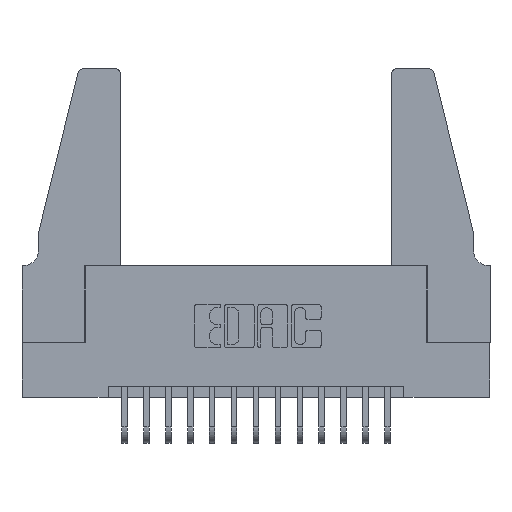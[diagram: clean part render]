
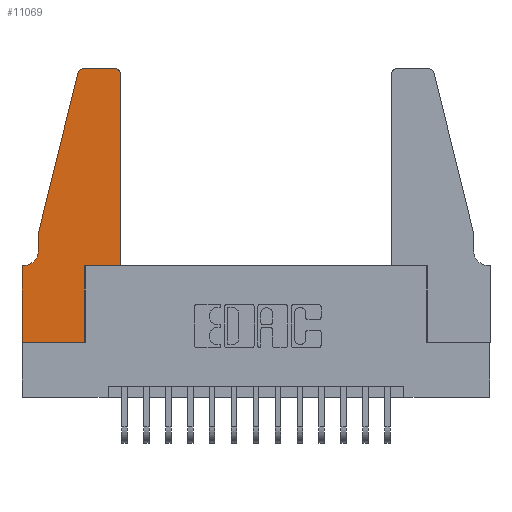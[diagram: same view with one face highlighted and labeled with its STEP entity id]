
A CAD part, top view. The second image highlights one B-rep face of the part: STEP entity #11069.
In plain terms, the highlighted planar face has unit normal (0, 0, 1).
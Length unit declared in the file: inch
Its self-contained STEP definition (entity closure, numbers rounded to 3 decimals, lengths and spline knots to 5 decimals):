
#33 = ORIENTED_EDGE ( 'NONE', *, *, #14486, .T. ) ;
#61 = ORIENTED_EDGE ( 'NONE', *, *, #15565, .T. ) ;
#193 = VECTOR ( 'NONE', #16897, 39.37008 ) ;
#360 = ORIENTED_EDGE ( 'NONE', *, *, #1850, .T. ) ;
#384 = ORIENTED_EDGE ( 'NONE', *, *, #16294, .T. ) ;
#399 = EDGE_CURVE ( 'NONE', #8588, #471, #10488, .T. ) ;
#471 = VERTEX_POINT ( 'NONE', #10095 ) ;
#742 = CARTESIAN_POINT ( 'NONE',  ( 0., 0., 0.37 ) ) ;
#871 = DIRECTION ( 'NONE',  ( 0., 1., 0. ) ) ;
#1189 = DIRECTION ( 'NONE',  ( 0., 0., 1. ) ) ;
#1526 = CARTESIAN_POINT ( 'NONE',  ( 0., 0.35, 0.37 ) ) ;
#1615 = AXIS2_PLACEMENT_3D ( 'NONE', #14819, #6514, #16186 ) ;
#1850 = EDGE_CURVE ( 'NONE', #10646, #14504, #8796, .T. ) ;
#1902 = DIRECTION ( 'NONE',  ( 0., 0., 1. ) ) ;
#2235 = ORIENTED_EDGE ( 'NONE', *, *, #17432, .T. ) ;
#2282 = CARTESIAN_POINT ( 'NONE',  ( 0.0755, 0.5, 0.37 ) ) ;
#2535 = VECTOR ( 'NONE', #4090, 39.37008 ) ;
#2539 = CARTESIAN_POINT ( 'NONE',  ( 0., 0.35, 0.37 ) ) ;
#2607 = VECTOR ( 'NONE', #9708, 39.37008 ) ;
#3409 = EDGE_CURVE ( 'NONE', #16824, #8174, #16703, .T. ) ;
#3674 = CARTESIAN_POINT ( 'NONE',  ( 0.4205, 1.25, 0.37 ) ) ;
#3901 = VERTEX_POINT ( 'NONE', #14414 ) ;
#3915 = LINE ( 'NONE', #5807, #193 ) ;
#3987 = EDGE_CURVE ( 'NONE', #14285, #3901, #17745, .T. ) ;
#4090 = DIRECTION ( 'NONE',  ( -1., 0., 0. ) ) ;
#4354 = CARTESIAN_POINT ( 'NONE',  ( 0.2605, 1.25, 0.37 ) ) ;
#4937 = LINE ( 'NONE', #5912, #8229 ) ;
#4979 = CARTESIAN_POINT ( 'NONE',  ( 0.0055, 0.42, 0.37 ) ) ;
#5387 = VERTEX_POINT ( 'NONE', #15960 ) ;
#5807 = CARTESIAN_POINT ( 'NONE',  ( 0.4505, 0.35, 0.37 ) ) ;
#5912 = CARTESIAN_POINT ( 'NONE',  ( 0.0755, 0.5, 0.37 ) ) ;
#6019 = VERTEX_POINT ( 'NONE', #15827 ) ;
#6081 = EDGE_CURVE ( 'NONE', #5387, #12691, #6676, .T. ) ;
#6375 = DIRECTION ( 'NONE',  ( -1., 0., 0. ) ) ;
#6514 = DIRECTION ( 'NONE',  ( 0., 0., 1. ) ) ;
#6676 = CIRCLE ( 'NONE', #14884, 0.07 ) ;
#6685 = LINE ( 'NONE', #8529, #16852 ) ;
#7845 = DIRECTION ( 'NONE',  ( -0.239, -0.971, 0. ) ) ;
#8174 = VERTEX_POINT ( 'NONE', #11318 ) ;
#8229 = VECTOR ( 'NONE', #17000, 39.37008 ) ;
#8529 = CARTESIAN_POINT ( 'NONE',  ( 0., 0., 0.37 ) ) ;
#8588 = VERTEX_POINT ( 'NONE', #3674 ) ;
#8796 = LINE ( 'NONE', #11422, #12051 ) ;
#8840 = CARTESIAN_POINT ( 'NONE',  ( 0.0055, 0.35, 0.37 ) ) ;
#9048 = ORIENTED_EDGE ( 'NONE', *, *, #17122, .T. ) ;
#9460 = ORIENTED_EDGE ( 'NONE', *, *, #6081, .T. ) ;
#9575 = PLANE ( 'NONE',  #15169 ) ;
#9708 = DIRECTION ( 'NONE',  ( -1., 0., 0. ) ) ;
#9977 = LINE ( 'NONE', #11017, #2535 ) ;
#10095 = CARTESIAN_POINT ( 'NONE',  ( 0.284, 1.25, 0.37 ) ) ;
#10109 = DIRECTION ( 'NONE',  ( 0., 1., 0. ) ) ;
#10285 = CARTESIAN_POINT ( 'NONE',  ( 0.4205, 1.22, 0.37 ) ) ;
#10317 = ORIENTED_EDGE ( 'NONE', *, *, #3409, .T. ) ;
#10386 = VERTEX_POINT ( 'NONE', #13328 ) ;
#10488 = LINE ( 'NONE', #4354, #2607 ) ;
#10528 = DIRECTION ( 'NONE',  ( 0., -1., 0. ) ) ;
#10646 = VERTEX_POINT ( 'NONE', #13889 ) ;
#10975 = DIRECTION ( 'NONE',  ( 1., 0., 0. ) ) ;
#11017 = CARTESIAN_POINT ( 'NONE',  ( 0.0755, 0.35, 0.37 ) ) ;
#11054 = EDGE_LOOP ( 'NONE', ( #16492, #16521, #10317, #9048, #9460, #2235, #17538, #16885, #33, #61, #360, #384 ) ) ;
#11069 = ADVANCED_FACE ( 'NONE', ( #13031 ), #9575, .T. ) ;
#11318 = CARTESIAN_POINT ( 'NONE',  ( 0.0755, 0.5, 0.37 ) ) ;
#11422 = CARTESIAN_POINT ( 'NONE',  ( 0.4505, 0.35, 0.37 ) ) ;
#11667 = DIRECTION ( 'NONE',  ( 1., 0., 0. ) ) ;
#12051 = VECTOR ( 'NONE', #10109, 39.37008 ) ;
#12691 = VERTEX_POINT ( 'NONE', #8840 ) ;
#13031 = FACE_OUTER_BOUND ( 'NONE', #11054, .T. ) ;
#13055 = VECTOR ( 'NONE', #7845, 39.37008 ) ;
#13328 = CARTESIAN_POINT ( 'NONE',  ( 0.2865, 0.35, 0.37 ) ) ;
#13377 = CARTESIAN_POINT ( 'NONE',  ( 0.4505, 1.22, 0.37 ) ) ;
#13402 = CIRCLE ( 'NONE', #1615, 0.03 ) ;
#13889 = CARTESIAN_POINT ( 'NONE',  ( 0.4505, 0.35, 0.37 ) ) ;
#14063 = DIRECTION ( 'NONE',  ( 1., 0., 0. ) ) ;
#14285 = VERTEX_POINT ( 'NONE', #1526 ) ;
#14376 = LINE ( 'NONE', #16084, #17590 ) ;
#14414 = CARTESIAN_POINT ( 'NONE',  ( 0., 0., 0.37 ) ) ;
#14486 = EDGE_CURVE ( 'NONE', #6019, #10386, #14376, .T. ) ;
#14504 = VERTEX_POINT ( 'NONE', #13377 ) ;
#14548 = VECTOR ( 'NONE', #10528, 39.37008 ) ;
#14694 = DIRECTION ( 'NONE',  ( 0., 0., -1. ) ) ;
#14744 = CIRCLE ( 'NONE', #17627, 0.03 ) ;
#14819 = CARTESIAN_POINT ( 'NONE',  ( 0.284, 1.22, 0.37 ) ) ;
#14884 = AXIS2_PLACEMENT_3D ( 'NONE', #4979, #14694, #6375 ) ;
#14925 = CARTESIAN_POINT ( 'NONE',  ( 0.25487, 1.22718, 0.37 ) ) ;
#15169 = AXIS2_PLACEMENT_3D ( 'NONE', #2539, #1189, #10975 ) ;
#15565 = EDGE_CURVE ( 'NONE', #10386, #10646, #3915, .T. ) ;
#15827 = CARTESIAN_POINT ( 'NONE',  ( 0.2865, 0., 0.37 ) ) ;
#15960 = CARTESIAN_POINT ( 'NONE',  ( 0.0755, 0.42, 0.37 ) ) ;
#16084 = CARTESIAN_POINT ( 'NONE',  ( 0.2865, 0.35, 0.37 ) ) ;
#16186 = DIRECTION ( 'NONE',  ( 1., 0., 0. ) ) ;
#16294 = EDGE_CURVE ( 'NONE', #14504, #8588, #14744, .T. ) ;
#16492 = ORIENTED_EDGE ( 'NONE', *, *, #399, .T. ) ;
#16521 = ORIENTED_EDGE ( 'NONE', *, *, #17876, .T. ) ;
#16703 = LINE ( 'NONE', #2282, #13055 ) ;
#16824 = VERTEX_POINT ( 'NONE', #14925 ) ;
#16852 = VECTOR ( 'NONE', #14063, 39.37008 ) ;
#16885 = ORIENTED_EDGE ( 'NONE', *, *, #17029, .T. ) ;
#16897 = DIRECTION ( 'NONE',  ( 1., 0., 0. ) ) ;
#17000 = DIRECTION ( 'NONE',  ( 0., -1., 0. ) ) ;
#17029 = EDGE_CURVE ( 'NONE', #3901, #6019, #6685, .T. ) ;
#17122 = EDGE_CURVE ( 'NONE', #8174, #5387, #4937, .T. ) ;
#17432 = EDGE_CURVE ( 'NONE', #12691, #14285, #9977, .T. ) ;
#17538 = ORIENTED_EDGE ( 'NONE', *, *, #3987, .T. ) ;
#17590 = VECTOR ( 'NONE', #871, 39.37008 ) ;
#17627 = AXIS2_PLACEMENT_3D ( 'NONE', #10285, #1902, #11667 ) ;
#17745 = LINE ( 'NONE', #742, #14548 ) ;
#17876 = EDGE_CURVE ( 'NONE', #471, #16824, #13402, .T. ) ;
